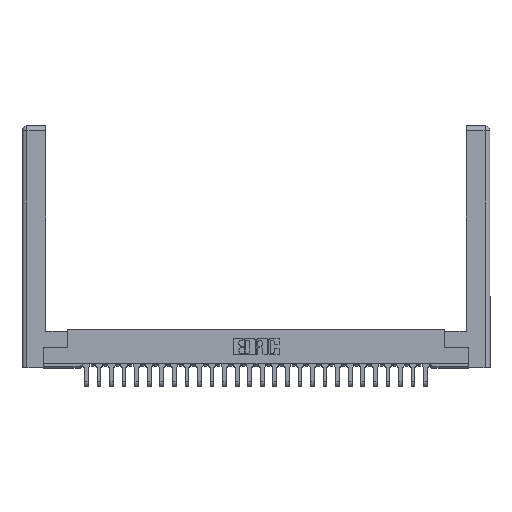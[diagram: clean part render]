
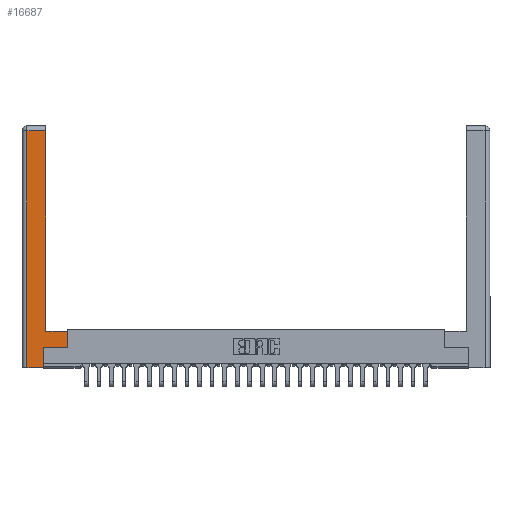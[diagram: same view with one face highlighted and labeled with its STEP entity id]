
A CAD part, top view. The second image highlights one B-rep face of the part: STEP entity #16687.
In plain terms, the highlighted planar face has unit normal (0, 0, 1).
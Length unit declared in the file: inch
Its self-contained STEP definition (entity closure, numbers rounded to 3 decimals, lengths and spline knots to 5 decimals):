
#556 = VECTOR ( 'NONE', #18537, 39.37008 ) ;
#1349 = CARTESIAN_POINT ( 'NONE',  ( 0.295, 0.45, 0. ) ) ;
#1740 = DIRECTION ( 'NONE',  ( -1., 0., 0. ) ) ;
#1823 = CARTESIAN_POINT ( 'NONE',  ( 0.265, 0., 0. ) ) ;
#2266 = EDGE_CURVE ( 'NONE', #13876, #29404, #14720, .T. ) ;
#2773 = CARTESIAN_POINT ( 'NONE',  ( 0.295, 2.94, 0. ) ) ;
#2874 = EDGE_CURVE ( 'NONE', #19669, #12588, #22726, .T. ) ;
#3580 = EDGE_CURVE ( 'NONE', #29404, #6515, #22305, .T. ) ;
#4372 = EDGE_CURVE ( 'NONE', #6515, #8377, #18843, .T. ) ;
#6238 = VERTEX_POINT ( 'NONE', #7113 ) ;
#6515 = VERTEX_POINT ( 'NONE', #18194 ) ;
#6599 = CARTESIAN_POINT ( 'NONE',  ( 0.0615, 0., 0. ) ) ;
#6628 = CARTESIAN_POINT ( 'NONE',  ( 0.265, 0., 0. ) ) ;
#6927 = LINE ( 'NONE', #9121, #20351 ) ;
#7113 = CARTESIAN_POINT ( 'NONE',  ( 0.265, 0.245, 0. ) ) ;
#8182 = AXIS2_PLACEMENT_3D ( 'NONE', #27268, #8185, #22120 ) ;
#8185 = DIRECTION ( 'NONE',  ( 0., 0., -1. ) ) ;
#8377 = VERTEX_POINT ( 'NONE', #6599 ) ;
#9121 = CARTESIAN_POINT ( 'NONE',  ( 0.565, 0.245, 0. ) ) ;
#9469 = DIRECTION ( 'NONE',  ( 0., 1., 0. ) ) ;
#10780 = DIRECTION ( 'NONE',  ( 0., 1., 0. ) ) ;
#11126 = LINE ( 'NONE', #1823, #29301 ) ;
#11336 = LINE ( 'NONE', #20819, #29632 ) ;
#11764 = ORIENTED_EDGE ( 'NONE', *, *, #3580, .T. ) ;
#11771 = CARTESIAN_POINT ( 'NONE',  ( 0.265, 0.245, 0. ) ) ;
#11981 = VECTOR ( 'NONE', #9469, 39.37008 ) ;
#12588 = VERTEX_POINT ( 'NONE', #29476 ) ;
#13106 = CARTESIAN_POINT ( 'NONE',  ( 0.565, 0.45, 0. ) ) ;
#13574 = ORIENTED_EDGE ( 'NONE', *, *, #4372, .T. ) ;
#13876 = VERTEX_POINT ( 'NONE', #1349 ) ;
#14720 = LINE ( 'NONE', #15170, #14869 ) ;
#14869 = VECTOR ( 'NONE', #19846, 39.37008 ) ;
#14878 = DIRECTION ( 'NONE',  ( -1., 0., 0. ) ) ;
#15170 = CARTESIAN_POINT ( 'NONE',  ( 0.295, 3., 0. ) ) ;
#15309 = ORIENTED_EDGE ( 'NONE', *, *, #30418, .T. ) ;
#16203 = CARTESIAN_POINT ( 'NONE',  ( 0.0615, 0., 0. ) ) ;
#16687 = ADVANCED_FACE ( 'NONE', ( #29465 ), #26967, .F. ) ;
#16897 = VECTOR ( 'NONE', #14878, 39.37008 ) ;
#17901 = ORIENTED_EDGE ( 'NONE', *, *, #2266, .T. ) ;
#18194 = CARTESIAN_POINT ( 'NONE',  ( 0.0615, 2.94, 0. ) ) ;
#18287 = EDGE_CURVE ( 'NONE', #6238, #19669, #6927, .T. ) ;
#18411 = EDGE_CURVE ( 'NONE', #8377, #23402, #11126, .T. ) ;
#18537 = DIRECTION ( 'NONE',  ( 0., -1., 0. ) ) ;
#18551 = DIRECTION ( 'NONE',  ( 1., 0., 0. ) ) ;
#18843 = LINE ( 'NONE', #16203, #556 ) ;
#19669 = VERTEX_POINT ( 'NONE', #23928 ) ;
#19846 = DIRECTION ( 'NONE',  ( 0., 1., 0. ) ) ;
#20351 = VECTOR ( 'NONE', #18551, 39.37008 ) ;
#20819 = CARTESIAN_POINT ( 'NONE',  ( 0.295, 0.45, 0. ) ) ;
#21096 = LINE ( 'NONE', #11771, #11981 ) ;
#21363 = EDGE_CURVE ( 'NONE', #23402, #6238, #21096, .T. ) ;
#22120 = DIRECTION ( 'NONE',  ( -1., 0., 0. ) ) ;
#22305 = LINE ( 'NONE', #26691, #16897 ) ;
#22726 = LINE ( 'NONE', #13106, #26314 ) ;
#23085 = DIRECTION ( 'NONE',  ( 1., 0., 0. ) ) ;
#23402 = VERTEX_POINT ( 'NONE', #6628 ) ;
#23928 = CARTESIAN_POINT ( 'NONE',  ( 0.565, 0.245, 0. ) ) ;
#23988 = EDGE_LOOP ( 'NONE', ( #17901, #11764, #13574, #28667, #24752, #28360, #27535, #15309 ) ) ;
#24752 = ORIENTED_EDGE ( 'NONE', *, *, #21363, .T. ) ;
#26314 = VECTOR ( 'NONE', #10780, 39.37008 ) ;
#26691 = CARTESIAN_POINT ( 'NONE',  ( 0.0615, 2.94, 0. ) ) ;
#26967 = PLANE ( 'NONE',  #8182 ) ;
#27268 = CARTESIAN_POINT ( 'NONE',  ( 0., 0., 0. ) ) ;
#27535 = ORIENTED_EDGE ( 'NONE', *, *, #2874, .T. ) ;
#28360 = ORIENTED_EDGE ( 'NONE', *, *, #18287, .T. ) ;
#28667 = ORIENTED_EDGE ( 'NONE', *, *, #18411, .T. ) ;
#29301 = VECTOR ( 'NONE', #23085, 39.37008 ) ;
#29404 = VERTEX_POINT ( 'NONE', #2773 ) ;
#29465 = FACE_OUTER_BOUND ( 'NONE', #23988, .T. ) ;
#29476 = CARTESIAN_POINT ( 'NONE',  ( 0.565, 0.45, 0. ) ) ;
#29632 = VECTOR ( 'NONE', #1740, 39.37008 ) ;
#30418 = EDGE_CURVE ( 'NONE', #12588, #13876, #11336, .T. ) ;
